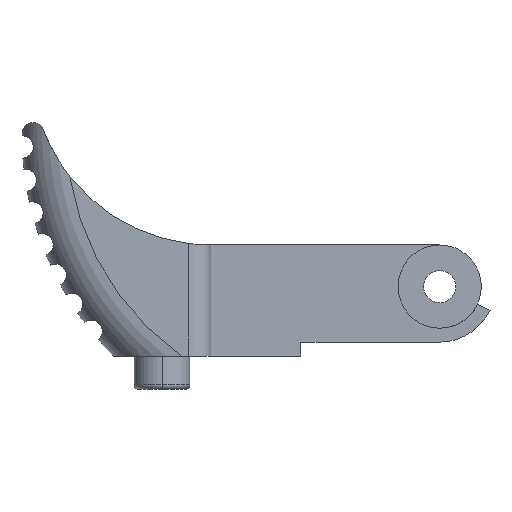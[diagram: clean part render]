
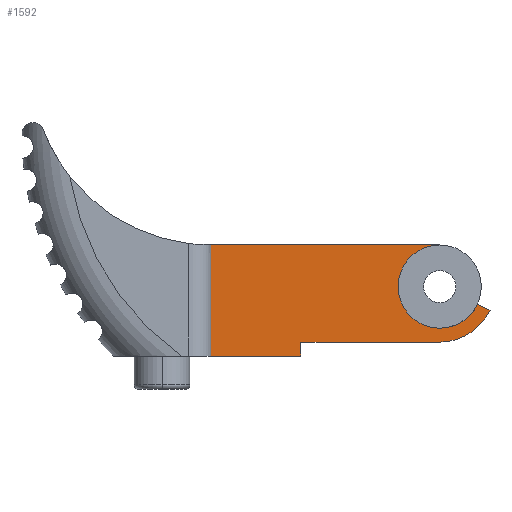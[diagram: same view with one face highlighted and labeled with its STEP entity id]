
A CAD part, left-side view. The second image highlights one B-rep face of the part: STEP entity #1592.
In plain terms, the highlighted planar face has unit normal (-1, 0, 0).
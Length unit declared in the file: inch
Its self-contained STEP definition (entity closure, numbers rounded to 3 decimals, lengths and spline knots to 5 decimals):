
#26 = EDGE_CURVE ( 'NONE', #1507, #521, #500, .T. ) ;
#31 = CARTESIAN_POINT ( 'NONE',  ( -0.125, 0., -0.25 ) ) ;
#55 = CARTESIAN_POINT ( 'NONE',  ( -0.125, 1.03, -0.313 ) ) ;
#69 = EDGE_CURVE ( 'NONE', #521, #1204, #1252, .T. ) ;
#70 = AXIS2_PLACEMENT_3D ( 'NONE', #1003, #843, #862 ) ;
#107 = LINE ( 'NONE', #1453, #483 ) ;
#197 = DIRECTION ( 'NONE',  ( 0., 1., 0. ) ) ;
#217 = EDGE_CURVE ( 'NONE', #1204, #374, #967, .T. ) ;
#345 = ORIENTED_EDGE ( 'NONE', *, *, #217, .F. ) ;
#355 = CARTESIAN_POINT ( 'NONE',  ( -0.125, 1.02936, 0.1875 ) ) ;
#374 = VERTEX_POINT ( 'NONE', #703 ) ;
#387 = CARTESIAN_POINT ( 'NONE',  ( -0.125, 0., 0.1875 ) ) ;
#404 = AXIS2_PLACEMENT_3D ( 'NONE', #1739, #844, #1890 ) ;
#416 = LINE ( 'NONE', #1169, #790 ) ;
#417 = CARTESIAN_POINT ( 'NONE',  ( -0.125, 1.03, -0.35 ) ) ;
#445 = CARTESIAN_POINT ( 'NONE',  ( -0.125, 1.03, -0.35 ) ) ;
#465 = ORIENTED_EDGE ( 'NONE', *, *, #664, .F. ) ;
#483 = VECTOR ( 'NONE', #197, 39.37008 ) ;
#500 = CIRCLE ( 'NONE', #70, 0.1875 ) ;
#502 = EDGE_CURVE ( 'NONE', #1267, #1862, #714, .T. ) ;
#521 = VERTEX_POINT ( 'NONE', #1968 ) ;
#558 = VECTOR ( 'NONE', #1316, 39.37008 ) ;
#571 = CARTESIAN_POINT ( 'NONE',  ( -0.125, -0.16993, -0.07924 ) ) ;
#575 = ORIENTED_EDGE ( 'NONE', *, *, #893, .F. ) ;
#610 = LINE ( 'NONE', #31, #558 ) ;
#620 = EDGE_LOOP ( 'NONE', ( #465, #1782, #1065, #1841, #575, #1190, #1843, #345, #969, #1329 ) ) ;
#635 = LINE ( 'NONE', #1727, #1417 ) ;
#656 = VECTOR ( 'NONE', #1533, 39.37008 ) ;
#664 = EDGE_CURVE ( 'NONE', #1253, #1507, #842, .T. ) ;
#671 = DIRECTION ( 'NONE',  ( 0., 0., -1. ) ) ;
#681 = EDGE_CURVE ( 'NONE', #770, #1319, #416, .T. ) ;
#699 = EDGE_CURVE ( 'NONE', #1862, #1046, #1599, .T. ) ;
#703 = CARTESIAN_POINT ( 'NONE',  ( -0.125, 0., -0.25 ) ) ;
#705 = CARTESIAN_POINT ( 'NONE',  ( -0.125, 1.02936, 0.99829 ) ) ;
#714 = LINE ( 'NONE', #445, #656 ) ;
#743 = CARTESIAN_POINT ( 'NONE',  ( -0.125, 1.03, 0.1875 ) ) ;
#770 = VERTEX_POINT ( 'NONE', #1133 ) ;
#790 = VECTOR ( 'NONE', #671, 39.37008 ) ;
#827 = DIRECTION ( 'NONE',  ( 0., -1., 0. ) ) ;
#842 = CIRCLE ( 'NONE', #404, 0.1875 ) ;
#843 = DIRECTION ( 'NONE',  ( -1., 0., 0. ) ) ;
#844 = DIRECTION ( 'NONE',  ( -1., 0., 0. ) ) ;
#849 = EDGE_CURVE ( 'NONE', #1046, #1253, #635, .T. ) ;
#862 = DIRECTION ( 'NONE',  ( 0., 1., 0. ) ) ;
#879 = DIRECTION ( 'NONE',  ( 0., 1., 0. ) ) ;
#893 = EDGE_CURVE ( 'NONE', #1319, #1267, #107, .T. ) ;
#899 = DIRECTION ( 'NONE',  ( 0., -0.906, -0.423 ) ) ;
#967 = CIRCLE ( 'NONE', #1124, 0.25 ) ;
#969 = ORIENTED_EDGE ( 'NONE', *, *, #69, .F. ) ;
#1003 = CARTESIAN_POINT ( 'NONE',  ( -0.125, 0., 0. ) ) ;
#1046 = VERTEX_POINT ( 'NONE', #355 ) ;
#1056 = EDGE_CURVE ( 'NONE', #374, #770, #610, .T. ) ;
#1065 = ORIENTED_EDGE ( 'NONE', *, *, #699, .F. ) ;
#1066 = CARTESIAN_POINT ( 'NONE',  ( -0.125, 0., -0.1875 ) ) ;
#1124 = AXIS2_PLACEMENT_3D ( 'NONE', #1799, #1807, #1936 ) ;
#1133 = CARTESIAN_POINT ( 'NONE',  ( -0.125, 0.625, -0.25 ) ) ;
#1169 = CARTESIAN_POINT ( 'NONE',  ( -0.125, 0.625, -0.25 ) ) ;
#1189 = CARTESIAN_POINT ( 'NONE',  ( -0.125, -0.22658, -0.10565 ) ) ;
#1190 = ORIENTED_EDGE ( 'NONE', *, *, #681, .F. ) ;
#1196 = CARTESIAN_POINT ( 'NONE',  ( -0.125, 0.625, -0.313 ) ) ;
#1204 = VERTEX_POINT ( 'NONE', #1189 ) ;
#1212 = VECTOR ( 'NONE', #899, 39.37008 ) ;
#1252 = LINE ( 'NONE', #571, #1212 ) ;
#1253 = VERTEX_POINT ( 'NONE', #387 ) ;
#1267 = VERTEX_POINT ( 'NONE', #55 ) ;
#1316 = DIRECTION ( 'NONE',  ( 0., 1., 0. ) ) ;
#1319 = VERTEX_POINT ( 'NONE', #1196 ) ;
#1329 = ORIENTED_EDGE ( 'NONE', *, *, #26, .F. ) ;
#1340 = AXIS2_PLACEMENT_3D ( 'NONE', #417, #1496, #1803 ) ;
#1417 = VECTOR ( 'NONE', #827, 39.37008 ) ;
#1453 = CARTESIAN_POINT ( 'NONE',  ( -0.125, 1.25, -0.313 ) ) ;
#1487 = FACE_OUTER_BOUND ( 'NONE', #620, .T. ) ;
#1496 = DIRECTION ( 'NONE',  ( 1., 0., 0. ) ) ;
#1507 = VERTEX_POINT ( 'NONE', #1066 ) ;
#1533 = DIRECTION ( 'NONE',  ( 0., 0., 1. ) ) ;
#1592 = ADVANCED_FACE ( 'NONE', ( #1487 ), #1652, .F. ) ;
#1599 = CIRCLE ( 'NONE', #1947, 0.81079 ) ;
#1652 = PLANE ( 'NONE',  #1340 ) ;
#1727 = CARTESIAN_POINT ( 'NONE',  ( -0.125, 0., 0.1875 ) ) ;
#1739 = CARTESIAN_POINT ( 'NONE',  ( -0.125, 0., 0. ) ) ;
#1771 = DIRECTION ( 'NONE',  ( -1., 0., 0. ) ) ;
#1782 = ORIENTED_EDGE ( 'NONE', *, *, #849, .F. ) ;
#1799 = CARTESIAN_POINT ( 'NONE',  ( -0.125, 0., 0. ) ) ;
#1803 = DIRECTION ( 'NONE',  ( 0., 1., 0. ) ) ;
#1807 = DIRECTION ( 'NONE',  ( 1., 0., 0. ) ) ;
#1841 = ORIENTED_EDGE ( 'NONE', *, *, #502, .F. ) ;
#1843 = ORIENTED_EDGE ( 'NONE', *, *, #1056, .F. ) ;
#1862 = VERTEX_POINT ( 'NONE', #743 ) ;
#1890 = DIRECTION ( 'NONE',  ( 0., 1., 0. ) ) ;
#1936 = DIRECTION ( 'NONE',  ( 0., 1., 0. ) ) ;
#1947 = AXIS2_PLACEMENT_3D ( 'NONE', #705, #1771, #879 ) ;
#1968 = CARTESIAN_POINT ( 'NONE',  ( -0.125, -0.16993, -0.07924 ) ) ;
